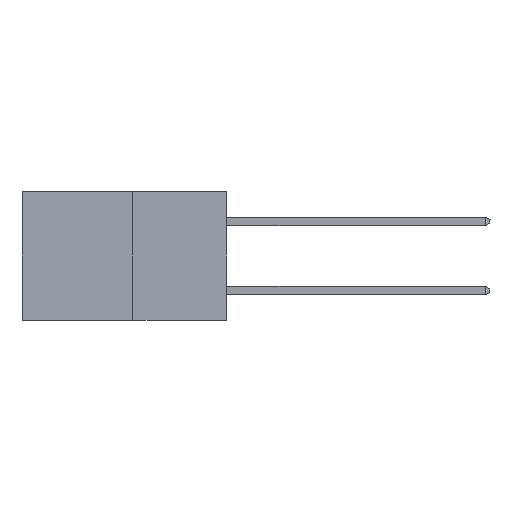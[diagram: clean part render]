
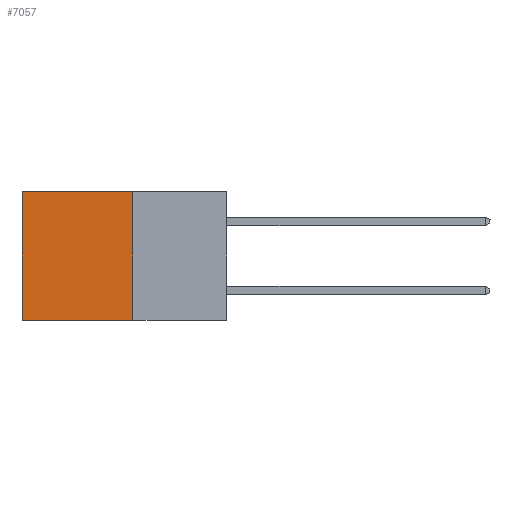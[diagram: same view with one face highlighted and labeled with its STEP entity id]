
A CAD part, left-side view. The second image highlights one B-rep face of the part: STEP entity #7057.
In plain terms, the highlighted planar face has unit normal (-1, 0, 0).
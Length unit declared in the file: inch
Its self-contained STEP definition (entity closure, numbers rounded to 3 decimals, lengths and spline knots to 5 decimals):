
#525 = VERTEX_POINT ( 'NONE', #3904 ) ;
#553 = ORIENTED_EDGE ( 'NONE', *, *, #4977, .F. ) ;
#1102 = VECTOR ( 'NONE', #3888, 39.37008 ) ;
#1307 = LINE ( 'NONE', #7266, #8826 ) ;
#1470 = LINE ( 'NONE', #8072, #1102 ) ;
#1614 = AXIS2_PLACEMENT_3D ( 'NONE', #4683, #5765, #12782 ) ;
#2258 = DIRECTION ( 'NONE',  ( 0., 1., 0. ) ) ;
#3888 = DIRECTION ( 'NONE',  ( 0., 0., -1. ) ) ;
#3904 = CARTESIAN_POINT ( 'NONE',  ( 0.277, 0.59, -0.37 ) ) ;
#4040 = DIRECTION ( 'NONE',  ( 0., 0., -1. ) ) ;
#4054 = CARTESIAN_POINT ( 'NONE',  ( 0.277, 0.27, -0.37 ) ) ;
#4144 = EDGE_CURVE ( 'NONE', #7031, #525, #1307, .T. ) ;
#4683 = CARTESIAN_POINT ( 'NONE',  ( 0.277, 0.27, -0.37 ) ) ;
#4977 = EDGE_CURVE ( 'NONE', #5677, #525, #7973, .T. ) ;
#5677 = VERTEX_POINT ( 'NONE', #7574 ) ;
#5765 = DIRECTION ( 'NONE',  ( 1., 0., 0. ) ) ;
#6181 = VERTEX_POINT ( 'NONE', #6410 ) ;
#6410 = CARTESIAN_POINT ( 'NONE',  ( 0.277, 0.27, 0. ) ) ;
#6607 = EDGE_CURVE ( 'NONE', #6181, #5677, #1470, .T. ) ;
#7031 = VERTEX_POINT ( 'NONE', #12747 ) ;
#7057 = ADVANCED_FACE ( 'NONE', ( #11009 ), #10864, .F. ) ;
#7266 = CARTESIAN_POINT ( 'NONE',  ( 0.277, 0.59, -0.37 ) ) ;
#7574 = CARTESIAN_POINT ( 'NONE',  ( 0.277, 0.27, -0.37 ) ) ;
#7621 = CARTESIAN_POINT ( 'NONE',  ( 0.277, 0.27, 0. ) ) ;
#7973 = LINE ( 'NONE', #4054, #8297 ) ;
#8072 = CARTESIAN_POINT ( 'NONE',  ( 0.277, 0.27, -0.37 ) ) ;
#8297 = VECTOR ( 'NONE', #11282, 39.37008 ) ;
#8826 = VECTOR ( 'NONE', #4040, 39.37008 ) ;
#9243 = EDGE_CURVE ( 'NONE', #6181, #7031, #9398, .T. ) ;
#9341 = EDGE_LOOP ( 'NONE', ( #9757, #553, #10180, #10036 ) ) ;
#9398 = LINE ( 'NONE', #7621, #12031 ) ;
#9757 = ORIENTED_EDGE ( 'NONE', *, *, #4144, .T. ) ;
#10036 = ORIENTED_EDGE ( 'NONE', *, *, #9243, .T. ) ;
#10180 = ORIENTED_EDGE ( 'NONE', *, *, #6607, .F. ) ;
#10864 = PLANE ( 'NONE',  #1614 ) ;
#11009 = FACE_OUTER_BOUND ( 'NONE', #9341, .T. ) ;
#11282 = DIRECTION ( 'NONE',  ( 0., 1., 0. ) ) ;
#12031 = VECTOR ( 'NONE', #2258, 39.37008 ) ;
#12747 = CARTESIAN_POINT ( 'NONE',  ( 0.277, 0.59, 0. ) ) ;
#12782 = DIRECTION ( 'NONE',  ( 0., 0., -1. ) ) ;
